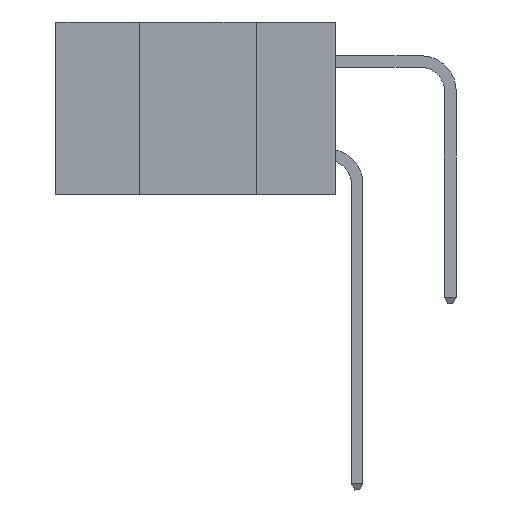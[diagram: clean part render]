
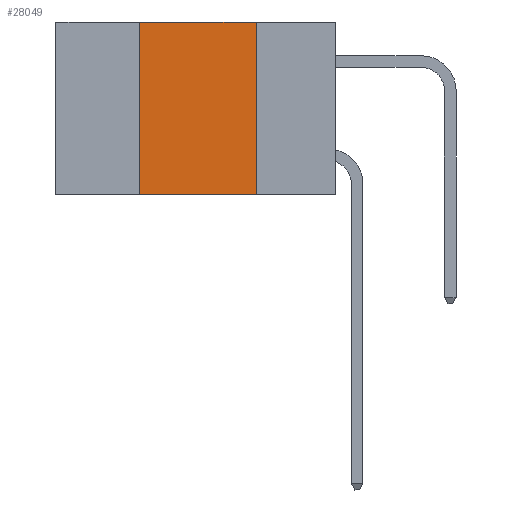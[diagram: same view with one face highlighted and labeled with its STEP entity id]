
A CAD part, left-side view. The second image highlights one B-rep face of the part: STEP entity #28049.
In plain terms, the highlighted planar face has unit normal (-1, 0, 0).
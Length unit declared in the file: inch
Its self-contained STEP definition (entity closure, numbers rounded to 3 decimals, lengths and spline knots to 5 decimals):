
#349 = CARTESIAN_POINT ( 'NONE',  ( 0., 0.17, -0.37 ) ) ;
#2841 = LINE ( 'NONE', #10601, #18116 ) ;
#3337 = VERTEX_POINT ( 'NONE', #27100 ) ;
#4178 = ORIENTED_EDGE ( 'NONE', *, *, #4872, .F. ) ;
#4872 = EDGE_CURVE ( 'NONE', #3337, #8598, #20694, .T. ) ;
#6131 = EDGE_CURVE ( 'NONE', #18112, #11280, #21387, .T. ) ;
#8444 = VECTOR ( 'NONE', #21801, 39.37008 ) ;
#8598 = VERTEX_POINT ( 'NONE', #349 ) ;
#8921 = CARTESIAN_POINT ( 'NONE',  ( 0., 0.42, 0. ) ) ;
#10149 = DIRECTION ( 'NONE',  ( 0., -1., 0. ) ) ;
#10601 = CARTESIAN_POINT ( 'NONE',  ( 0., 0.6, -0.37 ) ) ;
#11096 = PLANE ( 'NONE',  #26051 ) ;
#11280 = VERTEX_POINT ( 'NONE', #8921 ) ;
#12716 = CARTESIAN_POINT ( 'NONE',  ( 0., 0.6, 0. ) ) ;
#14838 = EDGE_CURVE ( 'NONE', #18112, #8598, #2841, .T. ) ;
#14927 = FACE_OUTER_BOUND ( 'NONE', #22904, .T. ) ;
#16331 = DIRECTION ( 'NONE',  ( 0., 0., 1. ) ) ;
#16505 = VECTOR ( 'NONE', #16331, 39.37008 ) ;
#17219 = EDGE_CURVE ( 'NONE', #11280, #3337, #22840, .T. ) ;
#18112 = VERTEX_POINT ( 'NONE', #21117 ) ;
#18116 = VECTOR ( 'NONE', #22708, 39.37008 ) ;
#18870 = CARTESIAN_POINT ( 'NONE',  ( 0., 0.42, 0. ) ) ;
#20638 = ORIENTED_EDGE ( 'NONE', *, *, #6131, .F. ) ;
#20694 = LINE ( 'NONE', #26442, #8444 ) ;
#21117 = CARTESIAN_POINT ( 'NONE',  ( 0., 0.42, -0.37 ) ) ;
#21387 = LINE ( 'NONE', #18870, #16505 ) ;
#21801 = DIRECTION ( 'NONE',  ( 0., 0., -1. ) ) ;
#22708 = DIRECTION ( 'NONE',  ( 0., -1., 0. ) ) ;
#22840 = LINE ( 'NONE', #12716, #29486 ) ;
#22904 = EDGE_LOOP ( 'NONE', ( #4178, #30639, #20638, #30129 ) ) ;
#25070 = DIRECTION ( 'NONE',  ( 0., 0., -1. ) ) ;
#26051 = AXIS2_PLACEMENT_3D ( 'NONE', #27573, #27459, #25070 ) ;
#26442 = CARTESIAN_POINT ( 'NONE',  ( 0., 0.17, 0. ) ) ;
#27100 = CARTESIAN_POINT ( 'NONE',  ( 0., 0.17, 0. ) ) ;
#27459 = DIRECTION ( 'NONE',  ( 1., 0., 0. ) ) ;
#27573 = CARTESIAN_POINT ( 'NONE',  ( 0., 0.6, 0. ) ) ;
#28049 = ADVANCED_FACE ( 'NONE', ( #14927 ), #11096, .F. ) ;
#29486 = VECTOR ( 'NONE', #10149, 39.37008 ) ;
#30129 = ORIENTED_EDGE ( 'NONE', *, *, #14838, .T. ) ;
#30639 = ORIENTED_EDGE ( 'NONE', *, *, #17219, .F. ) ;
